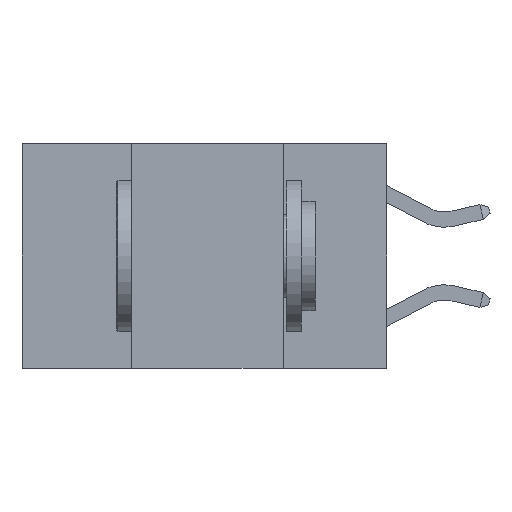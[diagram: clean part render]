
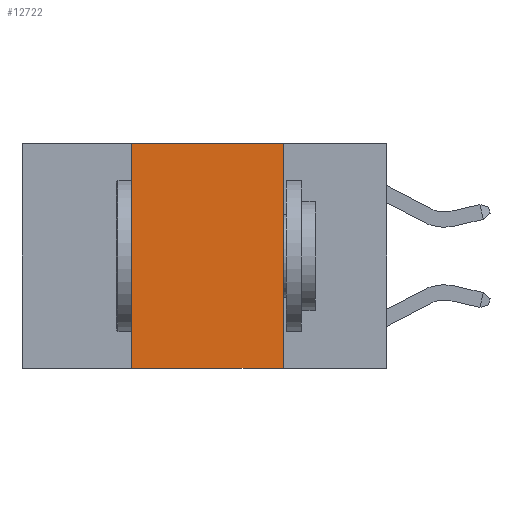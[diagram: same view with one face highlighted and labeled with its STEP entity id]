
A CAD part, left-side view. The second image highlights one B-rep face of the part: STEP entity #12722.
In plain terms, the highlighted planar face has unit normal (-1, 0, 0).
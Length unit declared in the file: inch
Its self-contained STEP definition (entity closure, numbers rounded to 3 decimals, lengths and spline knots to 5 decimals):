
#815 = ORIENTED_EDGE ( 'NONE', *, *, #4059, .F. ) ;
#3402 = LINE ( 'NONE', #8454, #14606 ) ;
#3467 = CARTESIAN_POINT ( 'NONE',  ( 0., 0.17, 0. ) ) ;
#4059 = EDGE_CURVE ( 'NONE', #13139, #13532, #9656, .T. ) ;
#4339 = DIRECTION ( 'NONE',  ( 1., 0., 0. ) ) ;
#4426 = CARTESIAN_POINT ( 'NONE',  ( 0., 0.6, 0. ) ) ;
#5818 = DIRECTION ( 'NONE',  ( 0., 0., -1. ) ) ;
#6702 = EDGE_CURVE ( 'NONE', #12238, #9817, #10981, .T. ) ;
#6774 = DIRECTION ( 'NONE',  ( 0., -1., 0. ) ) ;
#6906 = FACE_OUTER_BOUND ( 'NONE', #14239, .T. ) ;
#7200 = DIRECTION ( 'NONE',  ( 0., -1., 0. ) ) ;
#8077 = CARTESIAN_POINT ( 'NONE',  ( 0., 0.17, 0. ) ) ;
#8454 = CARTESIAN_POINT ( 'NONE',  ( 0., 0.6, 0. ) ) ;
#8492 = ORIENTED_EDGE ( 'NONE', *, *, #9561, .T. ) ;
#8520 = DIRECTION ( 'NONE',  ( 0., 0., -1. ) ) ;
#9312 = LINE ( 'NONE', #14638, #14608 ) ;
#9561 = EDGE_CURVE ( 'NONE', #13139, #9817, #9312, .T. ) ;
#9655 = VECTOR ( 'NONE', #8520, 39.37008 ) ;
#9656 = LINE ( 'NONE', #10851, #10593 ) ;
#9817 = VERTEX_POINT ( 'NONE', #9904 ) ;
#9848 = ORIENTED_EDGE ( 'NONE', *, *, #11298, .F. ) ;
#9879 = CARTESIAN_POINT ( 'NONE',  ( 0., 0.42, 0. ) ) ;
#9904 = CARTESIAN_POINT ( 'NONE',  ( 0., 0.17, -0.37 ) ) ;
#10494 = AXIS2_PLACEMENT_3D ( 'NONE', #4426, #4339, #5818 ) ;
#10593 = VECTOR ( 'NONE', #14728, 39.37008 ) ;
#10851 = CARTESIAN_POINT ( 'NONE',  ( 0., 0.42, 0. ) ) ;
#10981 = LINE ( 'NONE', #3467, #9655 ) ;
#11298 = EDGE_CURVE ( 'NONE', #13532, #12238, #3402, .T. ) ;
#11714 = CARTESIAN_POINT ( 'NONE',  ( 0., 0.42, -0.37 ) ) ;
#12042 = ORIENTED_EDGE ( 'NONE', *, *, #6702, .F. ) ;
#12238 = VERTEX_POINT ( 'NONE', #8077 ) ;
#12722 = ADVANCED_FACE ( 'NONE', ( #6906 ), #14753, .F. ) ;
#13139 = VERTEX_POINT ( 'NONE', #11714 ) ;
#13532 = VERTEX_POINT ( 'NONE', #9879 ) ;
#14239 = EDGE_LOOP ( 'NONE', ( #12042, #9848, #815, #8492 ) ) ;
#14606 = VECTOR ( 'NONE', #7200, 39.37008 ) ;
#14608 = VECTOR ( 'NONE', #6774, 39.37008 ) ;
#14638 = CARTESIAN_POINT ( 'NONE',  ( 0., 0.6, -0.37 ) ) ;
#14728 = DIRECTION ( 'NONE',  ( 0., 0., 1. ) ) ;
#14753 = PLANE ( 'NONE',  #10494 ) ;
